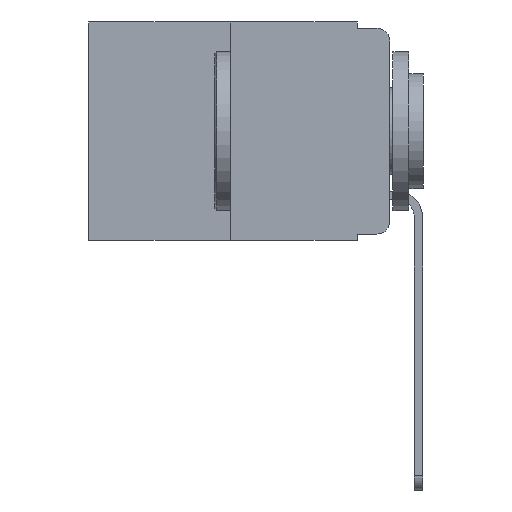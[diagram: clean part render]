
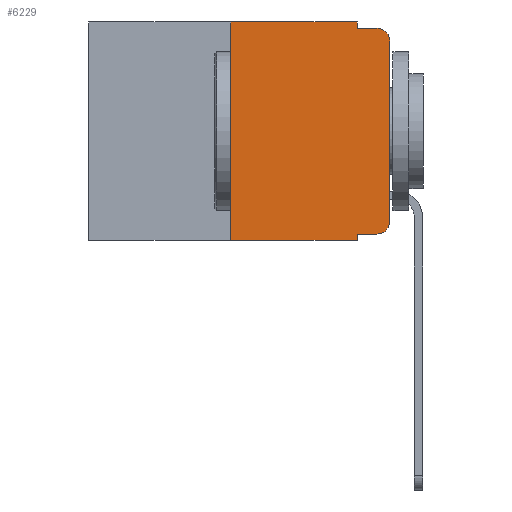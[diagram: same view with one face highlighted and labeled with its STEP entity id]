
A CAD part, left-side view. The second image highlights one B-rep face of the part: STEP entity #6229.
In plain terms, the highlighted planar face has unit normal (-1, 0, 0).
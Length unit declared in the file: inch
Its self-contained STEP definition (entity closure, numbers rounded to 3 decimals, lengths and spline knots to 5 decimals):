
#368 = EDGE_LOOP ( 'NONE', ( #3347, #9909, #6119, #10302, #5584, #7781, #410, #6959, #4522, #2423 ) ) ;
#410 = ORIENTED_EDGE ( 'NONE', *, *, #8859, .T. ) ;
#446 = CARTESIAN_POINT ( 'NONE',  ( 0., 0.25, 0. ) ) ;
#846 = CARTESIAN_POINT ( 'NONE',  ( 0., 0.473, 0. ) ) ;
#1083 = VERTEX_POINT ( 'NONE', #1736 ) ;
#1472 = VERTEX_POINT ( 'NONE', #2159 ) ;
#1736 = CARTESIAN_POINT ( 'NONE',  ( 0., 0., -0.313 ) ) ;
#2067 = CARTESIAN_POINT ( 'NONE',  ( 0., 0.25, -0.343 ) ) ;
#2159 = CARTESIAN_POINT ( 'NONE',  ( 0., 0.02, -0.333 ) ) ;
#2411 = VECTOR ( 'NONE', #9731, 39.37008 ) ;
#2413 = EDGE_CURVE ( 'NONE', #7564, #11127, #3191, .T. ) ;
#2423 = ORIENTED_EDGE ( 'NONE', *, *, #2939, .T. ) ;
#2491 = CARTESIAN_POINT ( 'NONE',  ( 0., 0.051, -0.01 ) ) ;
#2628 = FACE_OUTER_BOUND ( 'NONE', #368, .T. ) ;
#2730 = DIRECTION ( 'NONE',  ( 0., 0., -1. ) ) ;
#2868 = VERTEX_POINT ( 'NONE', #2491 ) ;
#2939 = EDGE_CURVE ( 'NONE', #1472, #1083, #5625, .T. ) ;
#3136 = CARTESIAN_POINT ( 'NONE',  ( 0., 0.473, 0. ) ) ;
#3174 = DIRECTION ( 'NONE',  ( 1., 0., 0. ) ) ;
#3175 = CARTESIAN_POINT ( 'NONE',  ( 0., 0.473, -0.343 ) ) ;
#3191 = CIRCLE ( 'NONE', #9539, 0.02 ) ;
#3347 = ORIENTED_EDGE ( 'NONE', *, *, #11112, .T. ) ;
#3836 = VERTEX_POINT ( 'NONE', #9044 ) ;
#3855 = DIRECTION ( 'NONE',  ( 0., 0., -1. ) ) ;
#3867 = DIRECTION ( 'NONE',  ( -1., 0., 0. ) ) ;
#3878 = CARTESIAN_POINT ( 'NONE',  ( 0., 0.02, -0.03 ) ) ;
#3900 = VECTOR ( 'NONE', #2730, 39.37008 ) ;
#4030 = LINE ( 'NONE', #846, #8693 ) ;
#4040 = DIRECTION ( 'NONE',  ( 0., -1., 0. ) ) ;
#4047 = VERTEX_POINT ( 'NONE', #8819 ) ;
#4174 = EDGE_CURVE ( 'NONE', #8449, #4047, #4030, .T. ) ;
#4358 = LINE ( 'NONE', #3175, #8753 ) ;
#4408 = CARTESIAN_POINT ( 'NONE',  ( 0., 0.02, -0.01 ) ) ;
#4431 = EDGE_CURVE ( 'NONE', #4047, #2868, #6215, .T. ) ;
#4522 = ORIENTED_EDGE ( 'NONE', *, *, #9972, .T. ) ;
#4747 = VECTOR ( 'NONE', #8844, 39.37008 ) ;
#4777 = LINE ( 'NONE', #10579, #2411 ) ;
#5244 = CARTESIAN_POINT ( 'NONE',  ( 0., 0., 0. ) ) ;
#5264 = CARTESIAN_POINT ( 'NONE',  ( 0., 0.02, -0.313 ) ) ;
#5403 = DIRECTION ( 'NONE',  ( 0., 0., -1. ) ) ;
#5485 = LINE ( 'NONE', #10566, #7559 ) ;
#5584 = ORIENTED_EDGE ( 'NONE', *, *, #4174, .F. ) ;
#5625 = CIRCLE ( 'NONE', #6362, 0.02 ) ;
#5716 = CARTESIAN_POINT ( 'NONE',  ( 0., 0.051, -0.343 ) ) ;
#6098 = VERTEX_POINT ( 'NONE', #2067 ) ;
#6119 = ORIENTED_EDGE ( 'NONE', *, *, #8555, .F. ) ;
#6129 = DIRECTION ( 'NONE',  ( 0., 0., 1. ) ) ;
#6201 = CARTESIAN_POINT ( 'NONE',  ( 0., 0.051, -0.333 ) ) ;
#6215 = LINE ( 'NONE', #11278, #3900 ) ;
#6229 = ADVANCED_FACE ( 'NONE', ( #2628 ), #8420, .F. ) ;
#6362 = AXIS2_PLACEMENT_3D ( 'NONE', #5264, #9735, #9714 ) ;
#6599 = VECTOR ( 'NONE', #6129, 39.37008 ) ;
#6816 = DIRECTION ( 'NONE',  ( 0., -1., 0. ) ) ;
#6959 = ORIENTED_EDGE ( 'NONE', *, *, #11257, .F. ) ;
#7287 = CARTESIAN_POINT ( 'NONE',  ( 0., 0., -0.03 ) ) ;
#7559 = VECTOR ( 'NONE', #5403, 39.37008 ) ;
#7564 = VERTEX_POINT ( 'NONE', #7287 ) ;
#7781 = ORIENTED_EDGE ( 'NONE', *, *, #10539, .F. ) ;
#7895 = CARTESIAN_POINT ( 'NONE',  ( 0., 0.25, 0. ) ) ;
#7992 = VECTOR ( 'NONE', #8621, 39.37008 ) ;
#8016 = AXIS2_PLACEMENT_3D ( 'NONE', #3136, #3174, #9250 ) ;
#8420 = PLANE ( 'NONE',  #8016 ) ;
#8449 = VERTEX_POINT ( 'NONE', #7895 ) ;
#8555 = EDGE_CURVE ( 'NONE', #2868, #11127, #4777, .T. ) ;
#8621 = DIRECTION ( 'NONE',  ( 0., 0., 1. ) ) ;
#8693 = VECTOR ( 'NONE', #6816, 39.37008 ) ;
#8753 = VECTOR ( 'NONE', #4040, 39.37008 ) ;
#8819 = CARTESIAN_POINT ( 'NONE',  ( 0., 0.051, 0. ) ) ;
#8844 = DIRECTION ( 'NONE',  ( 0., -1., 0. ) ) ;
#8859 = EDGE_CURVE ( 'NONE', #6098, #9620, #4358, .T. ) ;
#9044 = CARTESIAN_POINT ( 'NONE',  ( 0., 0.051, -0.333 ) ) ;
#9250 = DIRECTION ( 'NONE',  ( 0., 0., -1. ) ) ;
#9359 = LINE ( 'NONE', #6201, #4747 ) ;
#9539 = AXIS2_PLACEMENT_3D ( 'NONE', #3878, #3867, #3855 ) ;
#9620 = VERTEX_POINT ( 'NONE', #5716 ) ;
#9714 = DIRECTION ( 'NONE',  ( 0., 0., -1. ) ) ;
#9731 = DIRECTION ( 'NONE',  ( 0., -1., 0. ) ) ;
#9735 = DIRECTION ( 'NONE',  ( -1., 0., 0. ) ) ;
#9909 = ORIENTED_EDGE ( 'NONE', *, *, #2413, .T. ) ;
#9961 = LINE ( 'NONE', #446, #7992 ) ;
#9972 = EDGE_CURVE ( 'NONE', #3836, #1472, #9359, .T. ) ;
#10302 = ORIENTED_EDGE ( 'NONE', *, *, #4431, .F. ) ;
#10539 = EDGE_CURVE ( 'NONE', #6098, #8449, #9961, .T. ) ;
#10566 = CARTESIAN_POINT ( 'NONE',  ( 0., 0.051, 0. ) ) ;
#10579 = CARTESIAN_POINT ( 'NONE',  ( 0., 0.051, -0.01 ) ) ;
#11103 = LINE ( 'NONE', #5244, #6599 ) ;
#11112 = EDGE_CURVE ( 'NONE', #1083, #7564, #11103, .T. ) ;
#11127 = VERTEX_POINT ( 'NONE', #4408 ) ;
#11257 = EDGE_CURVE ( 'NONE', #3836, #9620, #5485, .T. ) ;
#11278 = CARTESIAN_POINT ( 'NONE',  ( 0., 0.051, 0. ) ) ;
